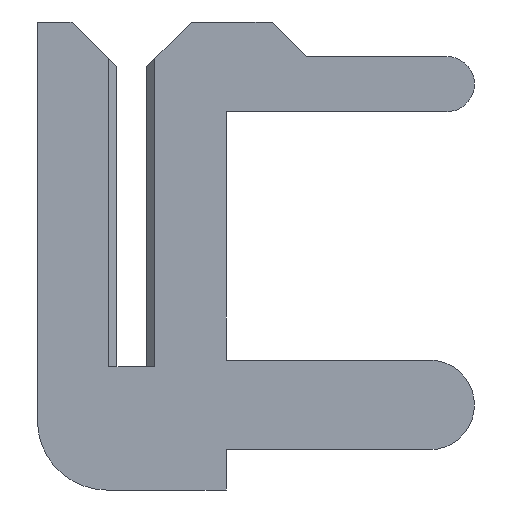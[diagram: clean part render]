
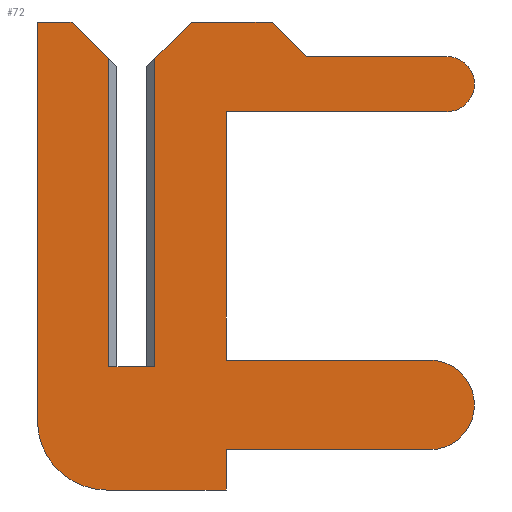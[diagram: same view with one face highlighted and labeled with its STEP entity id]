
A CAD part, left-side view. The second image highlights one B-rep face of the part: STEP entity #72.
In plain terms, the highlighted planar face has unit normal (-1, 0, 0).
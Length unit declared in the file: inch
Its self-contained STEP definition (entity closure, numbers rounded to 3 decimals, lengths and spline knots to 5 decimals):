
#5 = CARTESIAN_POINT ( 'NONE',  ( -0.01, -0.1295, 0.003 ) ) ;
#9 = CARTESIAN_POINT ( 'NONE',  ( -0.01, -0.137, 0.135 ) ) ;
#11 = ORIENTED_EDGE ( 'NONE', *, *, #578, .F. ) ;
#19 = DIRECTION ( 'NONE',  ( 0., 0., -1. ) ) ;
#36 = LINE ( 'NONE', #345, #1011 ) ;
#39 = CARTESIAN_POINT ( 'NONE',  ( -0.01, -0.0065, 0.1305 ) ) ;
#44 = LINE ( 'NONE', #708, #323 ) ;
#72 = ADVANCED_FACE ( 'NONE', ( #1222 ), #177, .T. ) ;
#73 = EDGE_CURVE ( 'NONE', #646, #991, #1130, .T. ) ;
#90 = EDGE_CURVE ( 'NONE', #485, #825, #982, .T. ) ;
#116 = CARTESIAN_POINT ( 'NONE',  ( -0.01, -0.137, 0.123 ) ) ;
#122 = ORIENTED_EDGE ( 'NONE', *, *, #1070, .F. ) ;
#159 = LINE ( 'NONE', #366, #1251 ) ;
#162 = CARTESIAN_POINT ( 'NONE',  ( -0.01, 0.041, -0.0235 ) ) ;
#177 = PLANE ( 'NONE',  #824 ) ;
#197 = CIRCLE ( 'NONE', #693, 0.012 ) ;
#205 = EDGE_CURVE ( 'NONE', #974, #431, #532, .T. ) ;
#208 = DIRECTION ( 'NONE',  ( 1., 0., 0. ) ) ;
#231 = DIRECTION ( 'NONE',  ( 0., -0.707, -0.707 ) ) ;
#237 = EDGE_CURVE ( 'NONE', #793, #485, #1054, .T. ) ;
#239 = ORIENTED_EDGE ( 'NONE', *, *, #645, .F. ) ;
#241 = VECTOR ( 'NONE', #1118, 39.37008 ) ;
#242 = CARTESIAN_POINT ( 'NONE',  ( -0.01, -0.041, 0.003 ) ) ;
#248 = VERTEX_POINT ( 'NONE', #328 ) ;
#258 = VECTOR ( 'NONE', #231, 39.37008 ) ;
#261 = CARTESIAN_POINT ( 'NONE',  ( -0.01, -0.076, 0.135 ) ) ;
#291 = ORIENTED_EDGE ( 'NONE', *, *, #329, .F. ) ;
#298 = DIRECTION ( 'NONE',  ( 0., -1., 0. ) ) ;
#303 = CARTESIAN_POINT ( 'NONE',  ( -0.01, -0.1295, -0.0165 ) ) ;
#308 = DIRECTION ( 'NONE',  ( 0., 0., -1. ) ) ;
#322 = EDGE_CURVE ( 'NONE', #1230, #646, #36, .T. ) ;
#323 = VECTOR ( 'NONE', #978, 39.37008 ) ;
#324 = VECTOR ( 'NONE', #298, 39.37008 ) ;
#328 = CARTESIAN_POINT ( 'NONE',  ( -0.01, 0.041, 0.15 ) ) ;
#329 = EDGE_CURVE ( 'NONE', #1061, #793, #489, .T. ) ;
#333 = DIRECTION ( 'NONE',  ( 0., -0.707, 0.707 ) ) ;
#345 = CARTESIAN_POINT ( 'NONE',  ( -0.01, -0.041, 0.111 ) ) ;
#350 = LINE ( 'NONE', #787, #1186 ) ;
#351 = VERTEX_POINT ( 'NONE', #162 ) ;
#366 = CARTESIAN_POINT ( 'NONE',  ( -0.01, 0.0065, 0. ) ) ;
#377 = CARTESIAN_POINT ( 'NONE',  ( -0.01, 0.026, 0.15 ) ) ;
#382 = DIRECTION ( 'NONE',  ( 0., 0., -1. ) ) ;
#394 = DIRECTION ( 'NONE',  ( 0., 1., 0. ) ) ;
#403 = CARTESIAN_POINT ( 'NONE',  ( -0.01, -0.041, -0.0535 ) ) ;
#412 = VECTOR ( 'NONE', #588, 39.37008 ) ;
#414 = CARTESIAN_POINT ( 'NONE',  ( -0.01, -0.137, 0.111 ) ) ;
#422 = CARTESIAN_POINT ( 'NONE',  ( -0.01, -0.01, 0.134 ) ) ;
#431 = VERTEX_POINT ( 'NONE', #261 ) ;
#444 = VECTOR ( 'NONE', #333, 39.37008 ) ;
#447 = CIRCLE ( 'NONE', #579, 0.03 ) ;
#450 = DIRECTION ( 'NONE',  ( 0., 1., 0. ) ) ;
#454 = VERTEX_POINT ( 'NONE', #647 ) ;
#467 = LINE ( 'NONE', #1000, #562 ) ;
#485 = VERTEX_POINT ( 'NONE', #661 ) ;
#488 = CARTESIAN_POINT ( 'NONE',  ( -0.01, -0.041, 0.111 ) ) ;
#489 = LINE ( 'NONE', #930, #241 ) ;
#494 = DIRECTION ( 'NONE',  ( 0., -0.707, -0.707 ) ) ;
#509 = VERTEX_POINT ( 'NONE', #764 ) ;
#512 = VECTOR ( 'NONE', #394, 39.37008 ) ;
#513 = DIRECTION ( 'NONE',  ( 0., 0., 1. ) ) ;
#523 = LINE ( 'NONE', #542, #412 ) ;
#532 = LINE ( 'NONE', #1180, #258 ) ;
#533 = CARTESIAN_POINT ( 'NONE',  ( -0.01, -0.061, 0.15 ) ) ;
#542 = CARTESIAN_POINT ( 'NONE',  ( -0.01, 0.026, 0.15 ) ) ;
#553 = ORIENTED_EDGE ( 'NONE', *, *, #1122, .T. ) ;
#554 = VERTEX_POINT ( 'NONE', #1240 ) ;
#562 = VECTOR ( 'NONE', #994, 39.37008 ) ;
#565 = ORIENTED_EDGE ( 'NONE', *, *, #685, .F. ) ;
#574 = CARTESIAN_POINT ( 'NONE',  ( -0.01, -0.041, 0.003 ) ) ;
#578 = EDGE_CURVE ( 'NONE', #703, #509, #159, .T. ) ;
#579 = AXIS2_PLACEMENT_3D ( 'NONE', #585, #208, #1072 ) ;
#585 = CARTESIAN_POINT ( 'NONE',  ( -0.01, 0.011, -0.0235 ) ) ;
#588 = DIRECTION ( 'NONE',  ( 0., -1., 0. ) ) ;
#610 = VECTOR ( 'NONE', #1203, 39.37008 ) ;
#621 = DIRECTION ( 'NONE',  ( 1., 0., 0. ) ) ;
#640 = ORIENTED_EDGE ( 'NONE', *, *, #1233, .T. ) ;
#642 = VERTEX_POINT ( 'NONE', #377 ) ;
#645 = EDGE_CURVE ( 'NONE', #825, #351, #447, .T. ) ;
#646 = VERTEX_POINT ( 'NONE', #488 ) ;
#647 = CARTESIAN_POINT ( 'NONE',  ( -0.01, 0.01, 0.134 ) ) ;
#661 = CARTESIAN_POINT ( 'NONE',  ( -0.01, -0.041, -0.0535 ) ) ;
#671 = LINE ( 'NONE', #1185, #1099 ) ;
#682 = LINE ( 'NONE', #9, #324 ) ;
#685 = EDGE_CURVE ( 'NONE', #706, #1061, #766, .T. ) ;
#691 = ORIENTED_EDGE ( 'NONE', *, *, #1210, .F. ) ;
#693 = AXIS2_PLACEMENT_3D ( 'NONE', #116, #621, #813 ) ;
#695 = CARTESIAN_POINT ( 'NONE',  ( -0.01, -0.041, -0.036 ) ) ;
#703 = VERTEX_POINT ( 'NONE', #1170 ) ;
#706 = VERTEX_POINT ( 'NONE', #5 ) ;
#708 = CARTESIAN_POINT ( 'NONE',  ( -0.01, -0.1295, 0.003 ) ) ;
#713 = EDGE_CURVE ( 'NONE', #431, #908, #682, .T. ) ;
#714 = AXIS2_PLACEMENT_3D ( 'NONE', #303, #859, #1064 ) ;
#735 = ORIENTED_EDGE ( 'NONE', *, *, #322, .F. ) ;
#741 = VECTOR ( 'NONE', #19, 39.37008 ) ;
#753 = EDGE_CURVE ( 'NONE', #908, #1230, #197, .T. ) ;
#764 = CARTESIAN_POINT ( 'NONE',  ( -0.01, -0.01, 0. ) ) ;
#766 = CIRCLE ( 'NONE', #714, 0.0195 ) ;
#787 = CARTESIAN_POINT ( 'NONE',  ( -0.01, 0.0065, 0.1305 ) ) ;
#793 = VERTEX_POINT ( 'NONE', #695 ) ;
#813 = DIRECTION ( 'NONE',  ( 0., 0., 1. ) ) ;
#815 = CARTESIAN_POINT ( 'NONE',  ( -0.01, -0.026, 0.15 ) ) ;
#824 = AXIS2_PLACEMENT_3D ( 'NONE', #1160, #1253, #1255 ) ;
#825 = VERTEX_POINT ( 'NONE', #1188 ) ;
#838 = ORIENTED_EDGE ( 'NONE', *, *, #713, .F. ) ;
#856 = ORIENTED_EDGE ( 'NONE', *, *, #237, .F. ) ;
#859 = DIRECTION ( 'NONE',  ( 1., 0., 0. ) ) ;
#871 = ORIENTED_EDGE ( 'NONE', *, *, #1204, .F. ) ;
#877 = CARTESIAN_POINT ( 'NONE',  ( -0.01, -0.137, 0.135 ) ) ;
#889 = ORIENTED_EDGE ( 'NONE', *, *, #1121, .F. ) ;
#908 = VERTEX_POINT ( 'NONE', #877 ) ;
#910 = ORIENTED_EDGE ( 'NONE', *, *, #73, .F. ) ;
#912 = VERTEX_POINT ( 'NONE', #422 ) ;
#930 = CARTESIAN_POINT ( 'NONE',  ( -0.01, -0.041, -0.036 ) ) ;
#953 = LINE ( 'NONE', #1093, #990 ) ;
#965 = EDGE_CURVE ( 'NONE', #554, #974, #1227, .T. ) ;
#974 = VERTEX_POINT ( 'NONE', #533 ) ;
#978 = DIRECTION ( 'NONE',  ( 0., -1., 0. ) ) ;
#981 = CARTESIAN_POINT ( 'NONE',  ( -0.01, 0.011, -0.0535 ) ) ;
#982 = LINE ( 'NONE', #981, #512 ) ;
#990 = VECTOR ( 'NONE', #308, 39.37008 ) ;
#991 = VERTEX_POINT ( 'NONE', #242 ) ;
#992 = EDGE_CURVE ( 'NONE', #912, #554, #1241, .T. ) ;
#994 = DIRECTION ( 'NONE',  ( 0., 0., 1. ) ) ;
#1000 = CARTESIAN_POINT ( 'NONE',  ( -0.01, 0.041, 0.15 ) ) ;
#1011 = VECTOR ( 'NONE', #450, 39.37008 ) ;
#1035 = ORIENTED_EDGE ( 'NONE', *, *, #753, .F. ) ;
#1053 = DIRECTION ( 'NONE',  ( 0., -1., 0. ) ) ;
#1054 = LINE ( 'NONE', #403, #741 ) ;
#1061 = VERTEX_POINT ( 'NONE', #1078 ) ;
#1064 = DIRECTION ( 'NONE',  ( 0., 0., 1. ) ) ;
#1070 = EDGE_CURVE ( 'NONE', #248, #642, #523, .T. ) ;
#1072 = DIRECTION ( 'NONE',  ( 0., 0., 1. ) ) ;
#1075 = ORIENTED_EDGE ( 'NONE', *, *, #90, .F. ) ;
#1078 = CARTESIAN_POINT ( 'NONE',  ( -0.01, -0.1295, -0.036 ) ) ;
#1082 = EDGE_LOOP ( 'NONE', ( #1193, #640, #11, #553, #889, #122, #691, #239, #1075, #856, #291, #565, #871, #910, #735, #1035, #838, #1164, #1181 ) ) ;
#1093 = CARTESIAN_POINT ( 'NONE',  ( -0.01, -0.01, 0.15 ) ) ;
#1099 = VECTOR ( 'NONE', #513, 39.37008 ) ;
#1118 = DIRECTION ( 'NONE',  ( 0., 1., 0. ) ) ;
#1121 = EDGE_CURVE ( 'NONE', #642, #454, #350, .T. ) ;
#1122 = EDGE_CURVE ( 'NONE', #703, #454, #671, .T. ) ;
#1130 = LINE ( 'NONE', #574, #1248 ) ;
#1160 = CARTESIAN_POINT ( 'NONE',  ( -0.01, 0.011, -0.0235 ) ) ;
#1164 = ORIENTED_EDGE ( 'NONE', *, *, #205, .F. ) ;
#1170 = CARTESIAN_POINT ( 'NONE',  ( -0.01, 0.01, 0. ) ) ;
#1180 = CARTESIAN_POINT ( 'NONE',  ( -0.01, -0.076, 0.135 ) ) ;
#1181 = ORIENTED_EDGE ( 'NONE', *, *, #965, .F. ) ;
#1185 = CARTESIAN_POINT ( 'NONE',  ( -0.01, 0.01, -0.0235 ) ) ;
#1186 = VECTOR ( 'NONE', #494, 39.37008 ) ;
#1188 = CARTESIAN_POINT ( 'NONE',  ( -0.01, 0.011, -0.0535 ) ) ;
#1193 = ORIENTED_EDGE ( 'NONE', *, *, #992, .F. ) ;
#1203 = DIRECTION ( 'NONE',  ( 0., -1., 0. ) ) ;
#1204 = EDGE_CURVE ( 'NONE', #991, #706, #44, .T. ) ;
#1210 = EDGE_CURVE ( 'NONE', #351, #248, #467, .T. ) ;
#1222 = FACE_OUTER_BOUND ( 'NONE', #1082, .T. ) ;
#1227 = LINE ( 'NONE', #815, #610 ) ;
#1230 = VERTEX_POINT ( 'NONE', #414 ) ;
#1233 = EDGE_CURVE ( 'NONE', #912, #509, #953, .T. ) ;
#1240 = CARTESIAN_POINT ( 'NONE',  ( -0.01, -0.026, 0.15 ) ) ;
#1241 = LINE ( 'NONE', #39, #444 ) ;
#1248 = VECTOR ( 'NONE', #382, 39.37008 ) ;
#1251 = VECTOR ( 'NONE', #1053, 39.37008 ) ;
#1253 = DIRECTION ( 'NONE',  ( -1., 0., 0. ) ) ;
#1255 = DIRECTION ( 'NONE',  ( 0., 0., 1. ) ) ;
